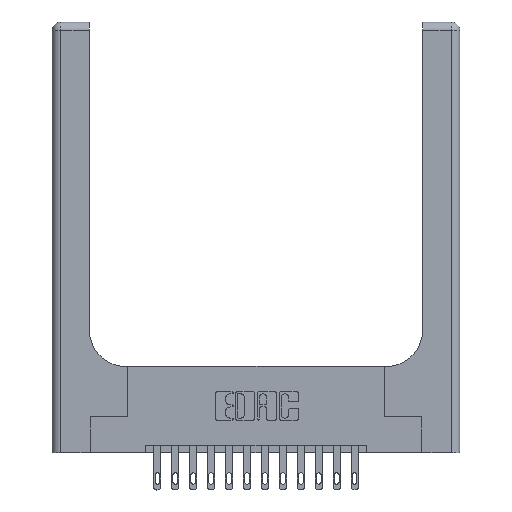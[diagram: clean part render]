
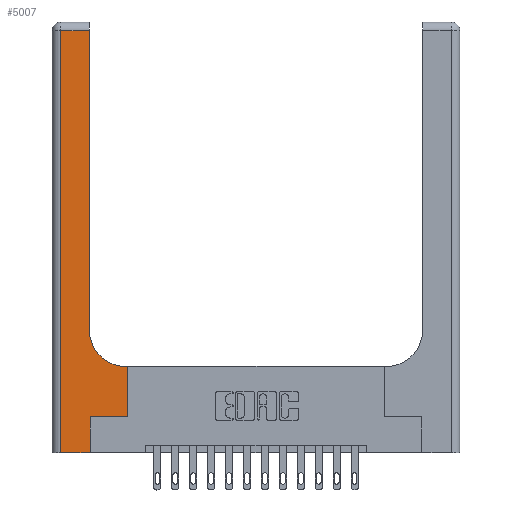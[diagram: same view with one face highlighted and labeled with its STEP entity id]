
A CAD part, top view. The second image highlights one B-rep face of the part: STEP entity #5007.
In plain terms, the highlighted planar face has unit normal (0, 0, 1).
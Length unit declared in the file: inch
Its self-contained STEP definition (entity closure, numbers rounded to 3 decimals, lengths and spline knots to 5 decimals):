
#170 = VERTEX_POINT ( 'NONE', #6455 ) ;
#503 = VERTEX_POINT ( 'NONE', #11321 ) ;
#575 = LINE ( 'NONE', #11375, #2978 ) ;
#617 = VERTEX_POINT ( 'NONE', #2981 ) ;
#654 = CARTESIAN_POINT ( 'NONE',  ( 0.26, 3., 0.37 ) ) ;
#766 = DIRECTION ( 'NONE',  ( -1., 0., 0. ) ) ;
#1203 = CARTESIAN_POINT ( 'NONE',  ( 0., 2.94, 0.37 ) ) ;
#1597 = VERTEX_POINT ( 'NONE', #16978 ) ;
#1797 = CARTESIAN_POINT ( 'NONE',  ( 0.26, 0.85, 0.37 ) ) ;
#1826 = CIRCLE ( 'NONE', #5555, 0.25 ) ;
#2022 = EDGE_CURVE ( 'NONE', #3614, #5238, #15189, .T. ) ;
#2293 = EDGE_CURVE ( 'NONE', #17260, #6400, #4607, .T. ) ;
#2306 = CARTESIAN_POINT ( 'NONE',  ( 0., 3., 0.37 ) ) ;
#2924 = VECTOR ( 'NONE', #9821, 39.37008 ) ;
#2959 = CARTESIAN_POINT ( 'NONE',  ( 0.528, 0.6, 0.37 ) ) ;
#2978 = VECTOR ( 'NONE', #15378, 39.37008 ) ;
#2981 = CARTESIAN_POINT ( 'NONE',  ( 0.265, 0.25, 0.37 ) ) ;
#3266 = CARTESIAN_POINT ( 'NONE',  ( 0.06, 3., 0.37 ) ) ;
#3352 = DIRECTION ( 'NONE',  ( 0., 1., 0. ) ) ;
#3614 = VERTEX_POINT ( 'NONE', #1797 ) ;
#3661 = LINE ( 'NONE', #15768, #10054 ) ;
#3716 = DIRECTION ( 'NONE',  ( 1., 0., 0. ) ) ;
#3829 = CARTESIAN_POINT ( 'NONE',  ( 0.26, 2.94, 0.37 ) ) ;
#4309 = VECTOR ( 'NONE', #3352, 39.37008 ) ;
#4607 = LINE ( 'NONE', #3266, #9956 ) ;
#4705 = EDGE_LOOP ( 'NONE', ( #7110, #8102, #15417, #8001, #11646, #10401, #7981, #14119, #14511 ) ) ;
#4788 = LINE ( 'NONE', #8492, #14220 ) ;
#5007 = ADVANCED_FACE ( 'NONE', ( #8960 ), #13025, .F. ) ;
#5035 = LINE ( 'NONE', #10419, #13789 ) ;
#5238 = VERTEX_POINT ( 'NONE', #3829 ) ;
#5329 = EDGE_CURVE ( 'NONE', #5238, #17260, #12040, .T. ) ;
#5555 = AXIS2_PLACEMENT_3D ( 'NONE', #6532, #7772, #6703 ) ;
#6041 = EDGE_CURVE ( 'NONE', #12890, #1597, #575, .T. ) ;
#6207 = AXIS2_PLACEMENT_3D ( 'NONE', #2306, #10530, #766 ) ;
#6400 = VERTEX_POINT ( 'NONE', #10864 ) ;
#6455 = CARTESIAN_POINT ( 'NONE',  ( 0.528, 0.25, 0.37 ) ) ;
#6532 = CARTESIAN_POINT ( 'NONE',  ( 0.51, 0.85, 0.37 ) ) ;
#6703 = DIRECTION ( 'NONE',  ( 1., 0., 0. ) ) ;
#6829 = CARTESIAN_POINT ( 'NONE',  ( 0.265, 0., 0.37 ) ) ;
#7110 = ORIENTED_EDGE ( 'NONE', *, *, #2022, .T. ) ;
#7431 = EDGE_CURVE ( 'NONE', #170, #12890, #3661, .T. ) ;
#7772 = DIRECTION ( 'NONE',  ( 0., 0., -1. ) ) ;
#7981 = ORIENTED_EDGE ( 'NONE', *, *, #7431, .T. ) ;
#8001 = ORIENTED_EDGE ( 'NONE', *, *, #13147, .T. ) ;
#8048 = DIRECTION ( 'NONE',  ( -1., 0., 0. ) ) ;
#8102 = ORIENTED_EDGE ( 'NONE', *, *, #5329, .T. ) ;
#8396 = LINE ( 'NONE', #6829, #2924 ) ;
#8492 = CARTESIAN_POINT ( 'NONE',  ( 0.265, 0.25, 0.37 ) ) ;
#8852 = DIRECTION ( 'NONE',  ( 1., 0., 0. ) ) ;
#8960 = FACE_OUTER_BOUND ( 'NONE', #4705, .T. ) ;
#9821 = DIRECTION ( 'NONE',  ( 0., 1., 0. ) ) ;
#9831 = EDGE_CURVE ( 'NONE', #1597, #3614, #1826, .T. ) ;
#9956 = VECTOR ( 'NONE', #11199, 39.37008 ) ;
#10054 = VECTOR ( 'NONE', #10532, 39.37008 ) ;
#10135 = EDGE_CURVE ( 'NONE', #617, #170, #4788, .T. ) ;
#10401 = ORIENTED_EDGE ( 'NONE', *, *, #10135, .T. ) ;
#10419 = CARTESIAN_POINT ( 'NONE',  ( 0., 0., 0.37 ) ) ;
#10530 = DIRECTION ( 'NONE',  ( 0., 0., -1. ) ) ;
#10532 = DIRECTION ( 'NONE',  ( 0., 1., 0. ) ) ;
#10864 = CARTESIAN_POINT ( 'NONE',  ( 0.06, 0., 0.37 ) ) ;
#11111 = CARTESIAN_POINT ( 'NONE',  ( 0.06, 2.94, 0.37 ) ) ;
#11199 = DIRECTION ( 'NONE',  ( 0., -1., 0. ) ) ;
#11321 = CARTESIAN_POINT ( 'NONE',  ( 0.265, 0., 0.37 ) ) ;
#11375 = CARTESIAN_POINT ( 'NONE',  ( 0.26, 0.6, 0.37 ) ) ;
#11646 = ORIENTED_EDGE ( 'NONE', *, *, #12323, .T. ) ;
#12040 = LINE ( 'NONE', #1203, #15138 ) ;
#12323 = EDGE_CURVE ( 'NONE', #503, #617, #8396, .T. ) ;
#12890 = VERTEX_POINT ( 'NONE', #2959 ) ;
#13025 = PLANE ( 'NONE',  #6207 ) ;
#13147 = EDGE_CURVE ( 'NONE', #6400, #503, #5035, .T. ) ;
#13789 = VECTOR ( 'NONE', #3716, 39.37008 ) ;
#14119 = ORIENTED_EDGE ( 'NONE', *, *, #6041, .T. ) ;
#14220 = VECTOR ( 'NONE', #8852, 39.37008 ) ;
#14511 = ORIENTED_EDGE ( 'NONE', *, *, #9831, .T. ) ;
#15138 = VECTOR ( 'NONE', #8048, 39.37008 ) ;
#15189 = LINE ( 'NONE', #654, #4309 ) ;
#15378 = DIRECTION ( 'NONE',  ( -1., 0., 0. ) ) ;
#15417 = ORIENTED_EDGE ( 'NONE', *, *, #2293, .T. ) ;
#15768 = CARTESIAN_POINT ( 'NONE',  ( 0.528, 0.25, 0.37 ) ) ;
#16978 = CARTESIAN_POINT ( 'NONE',  ( 0.51, 0.6, 0.37 ) ) ;
#17260 = VERTEX_POINT ( 'NONE', #11111 ) ;
